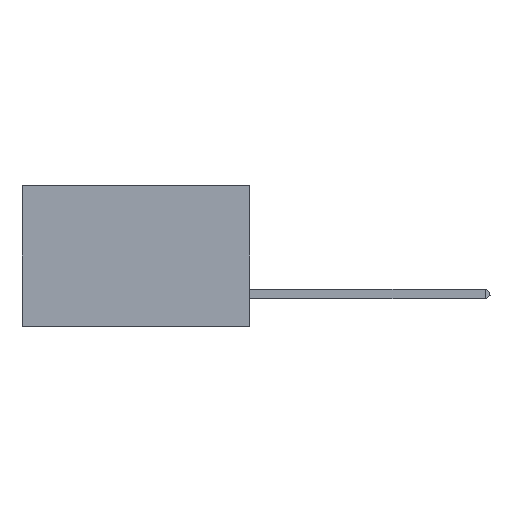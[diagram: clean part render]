
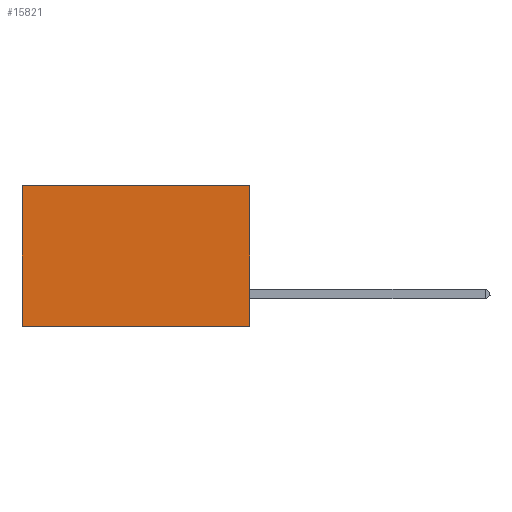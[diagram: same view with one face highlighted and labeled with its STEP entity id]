
A CAD part, left-side view. The second image highlights one B-rep face of the part: STEP entity #15821.
In plain terms, the highlighted planar face has unit normal (-1, 0, 0).
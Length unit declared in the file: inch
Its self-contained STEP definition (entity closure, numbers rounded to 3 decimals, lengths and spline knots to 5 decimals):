
#1640 = DIRECTION ( 'NONE',  ( 0., 1., 0. ) ) ;
#1675 = VERTEX_POINT ( 'NONE', #15914 ) ;
#2162 = DIRECTION ( 'NONE',  ( 0., 1., 0. ) ) ;
#2642 = ORIENTED_EDGE ( 'NONE', *, *, #15349, .T. ) ;
#4103 = CARTESIAN_POINT ( 'NONE',  ( 0.2875, 0., 0. ) ) ;
#4185 = ORIENTED_EDGE ( 'NONE', *, *, #5205, .T. ) ;
#5205 = EDGE_CURVE ( 'NONE', #11627, #21022, #11056, .T. ) ;
#6149 = ORIENTED_EDGE ( 'NONE', *, *, #24060, .F. ) ;
#6384 = DIRECTION ( 'NONE',  ( 0., 0., -1. ) ) ;
#8226 = VECTOR ( 'NONE', #1640, 39.37008 ) ;
#8586 = ORIENTED_EDGE ( 'NONE', *, *, #11910, .F. ) ;
#9712 = CARTESIAN_POINT ( 'NONE',  ( 0.2875, 0., 0. ) ) ;
#10156 = FACE_OUTER_BOUND ( 'NONE', #10406, .T. ) ;
#10406 = EDGE_LOOP ( 'NONE', ( #2642, #8586, #6149, #4185 ) ) ;
#11056 = LINE ( 'NONE', #9712, #11950 ) ;
#11627 = VERTEX_POINT ( 'NONE', #12417 ) ;
#11910 = EDGE_CURVE ( 'NONE', #1675, #14705, #13424, .T. ) ;
#11931 = CARTESIAN_POINT ( 'NONE',  ( 0.2875, 0.6, 0. ) ) ;
#11950 = VECTOR ( 'NONE', #2162, 39.37008 ) ;
#12417 = CARTESIAN_POINT ( 'NONE',  ( 0.2875, 0., 0. ) ) ;
#13424 = LINE ( 'NONE', #22888, #8226 ) ;
#13818 = LINE ( 'NONE', #11931, #17756 ) ;
#13905 = DIRECTION ( 'NONE',  ( 0., 0., -1. ) ) ;
#13981 = DIRECTION ( 'NONE',  ( 1., 0., 0. ) ) ;
#14705 = VERTEX_POINT ( 'NONE', #19509 ) ;
#15085 = DIRECTION ( 'NONE',  ( 0., 0., -1. ) ) ;
#15349 = EDGE_CURVE ( 'NONE', #21022, #14705, #13818, .T. ) ;
#15821 = ADVANCED_FACE ( 'NONE', ( #10156 ), #23647, .F. ) ;
#15914 = CARTESIAN_POINT ( 'NONE',  ( 0.2875, 0., -0.37 ) ) ;
#16962 = LINE ( 'NONE', #24652, #22395 ) ;
#17756 = VECTOR ( 'NONE', #6384, 39.37008 ) ;
#19509 = CARTESIAN_POINT ( 'NONE',  ( 0.2875, 0.6, -0.37 ) ) ;
#19727 = AXIS2_PLACEMENT_3D ( 'NONE', #4103, #13981, #13905 ) ;
#20380 = CARTESIAN_POINT ( 'NONE',  ( 0.2875, 0.6, 0. ) ) ;
#21022 = VERTEX_POINT ( 'NONE', #20380 ) ;
#22395 = VECTOR ( 'NONE', #15085, 39.37008 ) ;
#22888 = CARTESIAN_POINT ( 'NONE',  ( 0.2875, 0., -0.37 ) ) ;
#23647 = PLANE ( 'NONE',  #19727 ) ;
#24060 = EDGE_CURVE ( 'NONE', #11627, #1675, #16962, .T. ) ;
#24652 = CARTESIAN_POINT ( 'NONE',  ( 0.2875, 0., 0. ) ) ;
